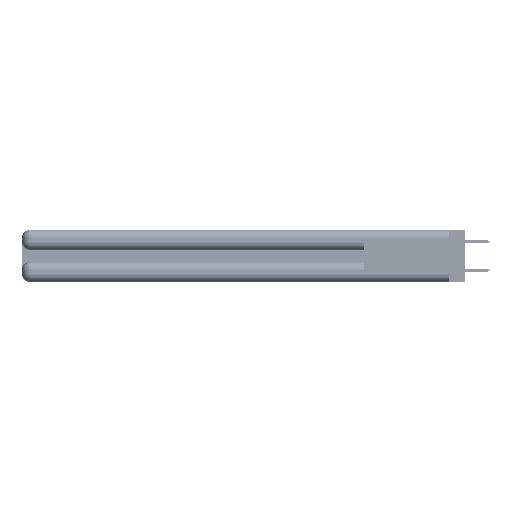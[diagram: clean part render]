
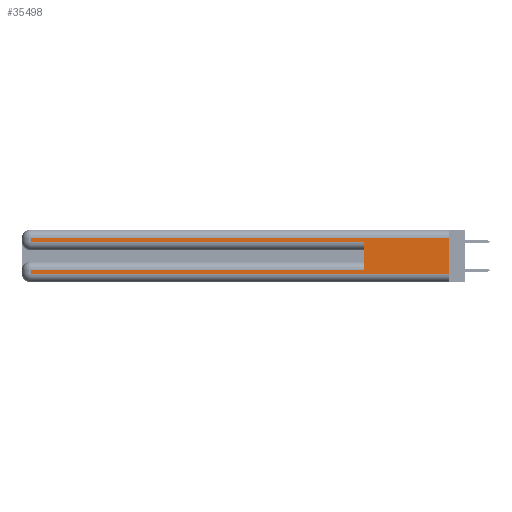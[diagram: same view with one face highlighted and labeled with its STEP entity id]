
A CAD part, left-side view. The second image highlights one B-rep face of the part: STEP entity #35498.
In plain terms, the highlighted planar face has unit normal (-1, 0, 0).
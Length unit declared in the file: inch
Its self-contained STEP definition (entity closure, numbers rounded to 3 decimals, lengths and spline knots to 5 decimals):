
#893 = LINE ( 'NONE', #14098, #36091 ) ;
#1296 = EDGE_CURVE ( 'NONE', #14593, #51337, #893, .T. ) ;
#1300 = LINE ( 'NONE', #35159, #31920 ) ;
#1868 = LINE ( 'NONE', #39022, #32494 ) ;
#3597 = CARTESIAN_POINT ( 'NONE',  ( 0., 0., 0.285 ) ) ;
#4212 = CARTESIAN_POINT ( 'NONE',  ( 0., 0.6, 0.285 ) ) ;
#5372 = CARTESIAN_POINT ( 'NONE',  ( 0., 0., 0.085 ) ) ;
#5969 = CARTESIAN_POINT ( 'NONE',  ( 0., 0.6, 0.145 ) ) ;
#6015 = DIRECTION ( 'NONE',  ( 0., 1., 0. ) ) ;
#6952 = LINE ( 'NONE', #5969, #16736 ) ;
#7164 = ORIENTED_EDGE ( 'NONE', *, *, #1296, .F. ) ;
#8457 = AXIS2_PLACEMENT_3D ( 'NONE', #13873, #42994, #18037 ) ;
#9451 = EDGE_CURVE ( 'NONE', #41543, #29974, #24600, .T. ) ;
#11123 = CARTESIAN_POINT ( 'NONE',  ( 0., 2.94, 0.31 ) ) ;
#13438 = DIRECTION ( 'NONE',  ( 0., -1., 0. ) ) ;
#13873 = CARTESIAN_POINT ( 'NONE',  ( 0., 0., 0.37 ) ) ;
#14098 = CARTESIAN_POINT ( 'NONE',  ( 0., 0., 0.37 ) ) ;
#14593 = VERTEX_POINT ( 'NONE', #20787 ) ;
#16187 = DIRECTION ( 'NONE',  ( 0., -1., 0. ) ) ;
#16736 = VECTOR ( 'NONE', #22555, 39.37008 ) ;
#17659 = VERTEX_POINT ( 'NONE', #11123 ) ;
#17918 = ORIENTED_EDGE ( 'NONE', *, *, #49523, .T. ) ;
#18037 = DIRECTION ( 'NONE',  ( 0., 0., -1. ) ) ;
#18777 = ORIENTED_EDGE ( 'NONE', *, *, #45257, .T. ) ;
#19926 = ORIENTED_EDGE ( 'NONE', *, *, #37941, .T. ) ;
#20787 = CARTESIAN_POINT ( 'NONE',  ( 0., 0., 0.31 ) ) ;
#21168 = LINE ( 'NONE', #43394, #51824 ) ;
#21231 = VECTOR ( 'NONE', #16187, 39.37008 ) ;
#22440 = DIRECTION ( 'NONE',  ( 0., 0., -1. ) ) ;
#22555 = DIRECTION ( 'NONE',  ( 0., 0., 1. ) ) ;
#24600 = LINE ( 'NONE', #5372, #47448 ) ;
#25098 = EDGE_LOOP ( 'NONE', ( #7164, #19926, #18777, #30379, #37722, #32916, #44118, #17918 ) ) ;
#25498 = EDGE_CURVE ( 'NONE', #41543, #44020, #6952, .T. ) ;
#26259 = CARTESIAN_POINT ( 'NONE',  ( 0., 0.6, 0.085 ) ) ;
#26819 = DIRECTION ( 'NONE',  ( 0., 0., -1. ) ) ;
#27929 = VERTEX_POINT ( 'NONE', #30934 ) ;
#29974 = VERTEX_POINT ( 'NONE', #30698 ) ;
#30379 = ORIENTED_EDGE ( 'NONE', *, *, #41860, .T. ) ;
#30698 = CARTESIAN_POINT ( 'NONE',  ( 0., 2.94, 0.085 ) ) ;
#30934 = CARTESIAN_POINT ( 'NONE',  ( 0., 2.94, 0.285 ) ) ;
#31124 = EDGE_CURVE ( 'NONE', #29974, #39962, #21168, .T. ) ;
#31920 = VECTOR ( 'NONE', #6015, 39.37008 ) ;
#32494 = VECTOR ( 'NONE', #26819, 39.37008 ) ;
#32916 = ORIENTED_EDGE ( 'NONE', *, *, #9451, .T. ) ;
#34948 = PLANE ( 'NONE',  #8457 ) ;
#35159 = CARTESIAN_POINT ( 'NONE',  ( 0., 0., 0.31 ) ) ;
#35498 = ADVANCED_FACE ( 'NONE', ( #49892 ), #34948, .F. ) ;
#36091 = VECTOR ( 'NONE', #22440, 39.37008 ) ;
#37722 = ORIENTED_EDGE ( 'NONE', *, *, #25498, .F. ) ;
#37941 = EDGE_CURVE ( 'NONE', #14593, #17659, #1300, .T. ) ;
#39022 = CARTESIAN_POINT ( 'NONE',  ( 0., 2.94, 0.37 ) ) ;
#39962 = VERTEX_POINT ( 'NONE', #45347 ) ;
#41543 = VERTEX_POINT ( 'NONE', #26259 ) ;
#41860 = EDGE_CURVE ( 'NONE', #27929, #44020, #42088, .T. ) ;
#41891 = VECTOR ( 'NONE', #13438, 39.37008 ) ;
#42088 = LINE ( 'NONE', #3597, #21231 ) ;
#42916 = DIRECTION ( 'NONE',  ( 0., 1., 0. ) ) ;
#42994 = DIRECTION ( 'NONE',  ( 1., 0., 0. ) ) ;
#43394 = CARTESIAN_POINT ( 'NONE',  ( 0., 2.94, 0.37 ) ) ;
#44020 = VERTEX_POINT ( 'NONE', #4212 ) ;
#44108 = DIRECTION ( 'NONE',  ( 0., 0., -1. ) ) ;
#44118 = ORIENTED_EDGE ( 'NONE', *, *, #31124, .T. ) ;
#45257 = EDGE_CURVE ( 'NONE', #17659, #27929, #1868, .T. ) ;
#45347 = CARTESIAN_POINT ( 'NONE',  ( 0., 2.94, 0.06 ) ) ;
#46053 = CARTESIAN_POINT ( 'NONE',  ( 0., 0., 0.06 ) ) ;
#47448 = VECTOR ( 'NONE', #42916, 39.37008 ) ;
#49523 = EDGE_CURVE ( 'NONE', #39962, #51337, #52983, .T. ) ;
#49805 = CARTESIAN_POINT ( 'NONE',  ( 0., 0., 0.06 ) ) ;
#49892 = FACE_OUTER_BOUND ( 'NONE', #25098, .T. ) ;
#51337 = VERTEX_POINT ( 'NONE', #49805 ) ;
#51824 = VECTOR ( 'NONE', #44108, 39.37008 ) ;
#52983 = LINE ( 'NONE', #46053, #41891 ) ;
